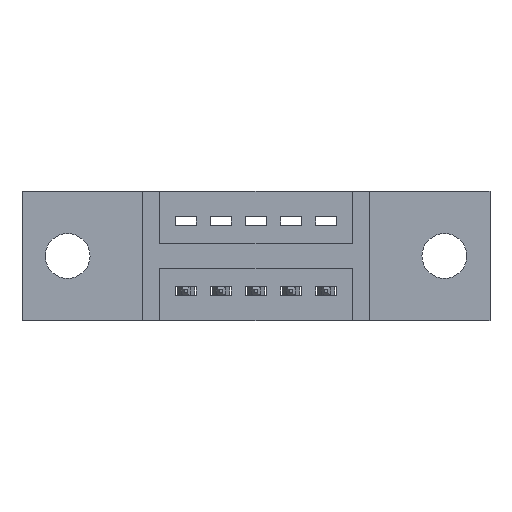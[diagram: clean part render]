
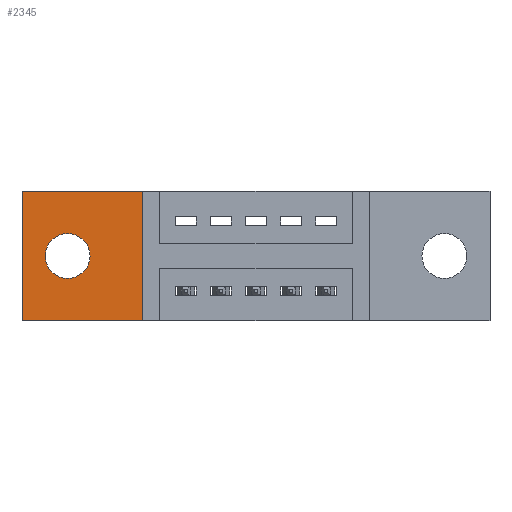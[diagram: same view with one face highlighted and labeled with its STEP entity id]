
A CAD part, front view. The second image highlights one B-rep face of the part: STEP entity #2345.
In plain terms, the highlighted planar face has unit normal (0, -1, 0).
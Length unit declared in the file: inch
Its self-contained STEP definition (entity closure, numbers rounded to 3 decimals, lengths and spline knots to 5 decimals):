
#90 = DIRECTION ( 'NONE',  ( 0., 0., -1. ) ) ;
#356 = EDGE_CURVE ( 'NONE', #8911, #4021, #3824, .T. ) ;
#362 = CIRCLE ( 'NONE', #2306, 0.064 ) ;
#694 = FACE_OUTER_BOUND ( 'NONE', #3668, .T. ) ;
#875 = ORIENTED_EDGE ( 'NONE', *, *, #4317, .T. ) ;
#1102 = CARTESIAN_POINT ( 'NONE',  ( 0., 0.11, -0.37 ) ) ;
#1288 = DIRECTION ( 'NONE',  ( 0., 0., 1. ) ) ;
#1533 = CARTESIAN_POINT ( 'NONE',  ( 0., 0.11, -0.37 ) ) ;
#1814 = CARTESIAN_POINT ( 'NONE',  ( 0., 0.11, 0. ) ) ;
#2238 = ORIENTED_EDGE ( 'NONE', *, *, #7789, .T. ) ;
#2259 = EDGE_CURVE ( 'NONE', #6497, #5286, #362, .T. ) ;
#2306 = AXIS2_PLACEMENT_3D ( 'NONE', #8080, #8044, #4593 ) ;
#2345 = ADVANCED_FACE ( 'NONE', ( #8319, #694 ), #6661, .T. ) ;
#2384 = LINE ( 'NONE', #1533, #6765 ) ;
#2554 = CIRCLE ( 'NONE', #6143, 0.064 ) ;
#2706 = ORIENTED_EDGE ( 'NONE', *, *, #3547, .T. ) ;
#3040 = CARTESIAN_POINT ( 'NONE',  ( 0.13, 0.11, -0.121 ) ) ;
#3395 = CARTESIAN_POINT ( 'NONE',  ( 0.13, 0.11, -0.185 ) ) ;
#3452 = LINE ( 'NONE', #7475, #8743 ) ;
#3547 = EDGE_CURVE ( 'NONE', #4021, #6534, #3452, .T. ) ;
#3668 = EDGE_LOOP ( 'NONE', ( #2238, #875, #5527, #2706 ) ) ;
#3824 = LINE ( 'NONE', #7419, #5223 ) ;
#3898 = DIRECTION ( 'NONE',  ( 0., 0., -1. ) ) ;
#3941 = ORIENTED_EDGE ( 'NONE', *, *, #2259, .F. ) ;
#4021 = VERTEX_POINT ( 'NONE', #4604 ) ;
#4078 = DIRECTION ( 'NONE',  ( -1., 0., 0. ) ) ;
#4124 = CARTESIAN_POINT ( 'NONE',  ( 0.3425, 0.11, -0.37 ) ) ;
#4244 = DIRECTION ( 'NONE',  ( 1., 0., 0. ) ) ;
#4317 = EDGE_CURVE ( 'NONE', #8117, #8911, #2384, .T. ) ;
#4474 = DIRECTION ( 'NONE',  ( 0., 0., -1. ) ) ;
#4593 = DIRECTION ( 'NONE',  ( 0., 0., -1. ) ) ;
#4604 = CARTESIAN_POINT ( 'NONE',  ( 0.3425, 0.11, 0. ) ) ;
#4845 = DIRECTION ( 'NONE',  ( 0., -1., 0. ) ) ;
#4962 = CARTESIAN_POINT ( 'NONE',  ( 0.13, 0.11, -0.249 ) ) ;
#5223 = VECTOR ( 'NONE', #1288, 39.37008 ) ;
#5286 = VERTEX_POINT ( 'NONE', #4962 ) ;
#5527 = ORIENTED_EDGE ( 'NONE', *, *, #356, .T. ) ;
#5663 = VECTOR ( 'NONE', #3898, 39.37008 ) ;
#5761 = LINE ( 'NONE', #1814, #5663 ) ;
#5889 = DIRECTION ( 'NONE',  ( 0., -1., 0. ) ) ;
#6011 = CARTESIAN_POINT ( 'NONE',  ( 0., 0.11, -0.37 ) ) ;
#6143 = AXIS2_PLACEMENT_3D ( 'NONE', #3395, #4845, #90 ) ;
#6413 = ORIENTED_EDGE ( 'NONE', *, *, #8906, .F. ) ;
#6497 = VERTEX_POINT ( 'NONE', #3040 ) ;
#6534 = VERTEX_POINT ( 'NONE', #8678 ) ;
#6661 = PLANE ( 'NONE',  #8011 ) ;
#6765 = VECTOR ( 'NONE', #4244, 39.37008 ) ;
#7419 = CARTESIAN_POINT ( 'NONE',  ( 0.3425, 0.11, 0. ) ) ;
#7475 = CARTESIAN_POINT ( 'NONE',  ( 0., 0.11, 0. ) ) ;
#7789 = EDGE_CURVE ( 'NONE', #6534, #8117, #5761, .T. ) ;
#8011 = AXIS2_PLACEMENT_3D ( 'NONE', #1102, #5889, #4474 ) ;
#8044 = DIRECTION ( 'NONE',  ( 0., -1., 0. ) ) ;
#8080 = CARTESIAN_POINT ( 'NONE',  ( 0.13, 0.11, -0.185 ) ) ;
#8117 = VERTEX_POINT ( 'NONE', #6011 ) ;
#8319 = FACE_BOUND ( 'NONE', #8488, .T. ) ;
#8488 = EDGE_LOOP ( 'NONE', ( #3941, #6413 ) ) ;
#8678 = CARTESIAN_POINT ( 'NONE',  ( 0., 0.11, 0. ) ) ;
#8743 = VECTOR ( 'NONE', #4078, 39.37008 ) ;
#8906 = EDGE_CURVE ( 'NONE', #5286, #6497, #2554, .T. ) ;
#8911 = VERTEX_POINT ( 'NONE', #4124 ) ;
